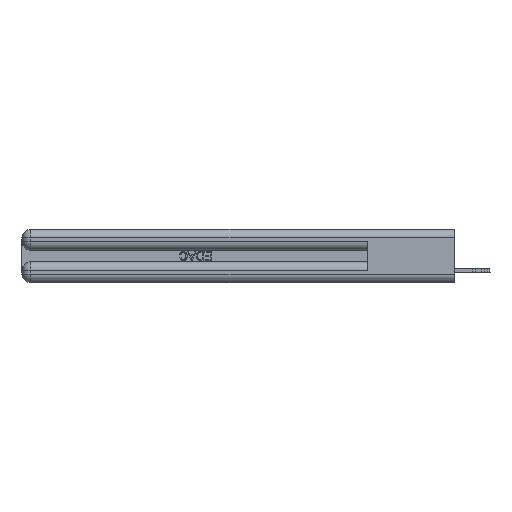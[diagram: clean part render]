
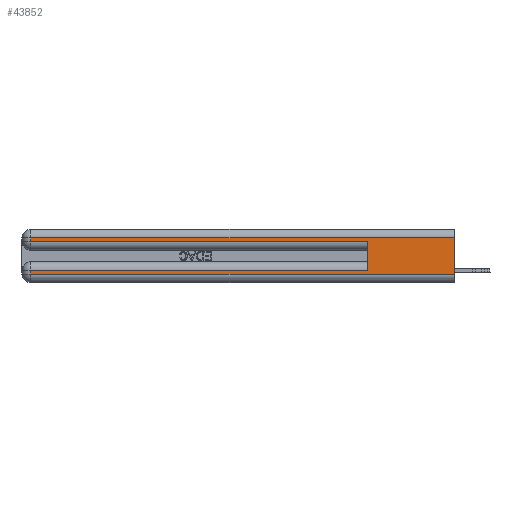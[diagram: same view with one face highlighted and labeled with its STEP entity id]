
A CAD part, left-side view. The second image highlights one B-rep face of the part: STEP entity #43852.
In plain terms, the highlighted planar face has unit normal (-1, 0, 0).
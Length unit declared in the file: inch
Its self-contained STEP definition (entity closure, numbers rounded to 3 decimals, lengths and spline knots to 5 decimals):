
#193 = VECTOR ( 'NONE', #38642, 39.37008 ) ;
#657 = VERTEX_POINT ( 'NONE', #24279 ) ;
#1644 = LINE ( 'NONE', #23310, #2255 ) ;
#1999 = VERTEX_POINT ( 'NONE', #6571 ) ;
#2255 = VECTOR ( 'NONE', #40804, 39.37008 ) ;
#2619 = ORIENTED_EDGE ( 'NONE', *, *, #31778, .T. ) ;
#2622 = VECTOR ( 'NONE', #15443, 39.37008 ) ;
#4887 = LINE ( 'NONE', #12556, #38072 ) ;
#5340 = EDGE_CURVE ( 'NONE', #1999, #20237, #39503, .T. ) ;
#5843 = ORIENTED_EDGE ( 'NONE', *, *, #5340, .T. ) ;
#6571 = CARTESIAN_POINT ( 'NONE',  ( 0., 2.94, 0.31 ) ) ;
#7212 = VERTEX_POINT ( 'NONE', #9270 ) ;
#8084 = LINE ( 'NONE', #36414, #35694 ) ;
#9270 = CARTESIAN_POINT ( 'NONE',  ( 0., 0., 0.06 ) ) ;
#10385 = AXIS2_PLACEMENT_3D ( 'NONE', #46592, #25127, #35892 ) ;
#10934 = DIRECTION ( 'NONE',  ( 0., 0., -1. ) ) ;
#12556 = CARTESIAN_POINT ( 'NONE',  ( 0., 0., 0.31 ) ) ;
#12734 = VERTEX_POINT ( 'NONE', #35527 ) ;
#13766 = LINE ( 'NONE', #38798, #193 ) ;
#14220 = PLANE ( 'NONE',  #10385 ) ;
#14344 = ORIENTED_EDGE ( 'NONE', *, *, #33568, .T. ) ;
#14900 = DIRECTION ( 'NONE',  ( 0., 1., 0. ) ) ;
#15334 = ORIENTED_EDGE ( 'NONE', *, *, #17748, .F. ) ;
#15363 = EDGE_CURVE ( 'NONE', #21128, #7212, #13766, .T. ) ;
#15443 = DIRECTION ( 'NONE',  ( 0., 0., -1. ) ) ;
#15903 = VECTOR ( 'NONE', #44245, 39.37008 ) ;
#17748 = EDGE_CURVE ( 'NONE', #12734, #657, #31736, .T. ) ;
#17859 = DIRECTION ( 'NONE',  ( 0., 0., 1. ) ) ;
#19142 = CARTESIAN_POINT ( 'NONE',  ( 0., 2.94, 0.37 ) ) ;
#20237 = VERTEX_POINT ( 'NONE', #33673 ) ;
#20327 = VECTOR ( 'NONE', #10934, 39.37008 ) ;
#20946 = EDGE_LOOP ( 'NONE', ( #27896, #14344, #5843, #44923, #15334, #2619, #46542, #33956 ) ) ;
#21128 = VERTEX_POINT ( 'NONE', #36643 ) ;
#22170 = VECTOR ( 'NONE', #17859, 39.37008 ) ;
#22489 = VERTEX_POINT ( 'NONE', #44840 ) ;
#23310 = CARTESIAN_POINT ( 'NONE',  ( 0., 0., 0.285 ) ) ;
#23622 = DIRECTION ( 'NONE',  ( 0., 1., 0. ) ) ;
#24279 = CARTESIAN_POINT ( 'NONE',  ( 0., 0.6, 0.285 ) ) ;
#25127 = DIRECTION ( 'NONE',  ( 1., 0., 0. ) ) ;
#25402 = CARTESIAN_POINT ( 'NONE',  ( 0., 0.6, 0.145 ) ) ;
#27673 = EDGE_CURVE ( 'NONE', #22489, #21128, #29817, .T. ) ;
#27896 = ORIENTED_EDGE ( 'NONE', *, *, #30560, .F. ) ;
#28928 = CARTESIAN_POINT ( 'NONE',  ( 0., 0., 0.31 ) ) ;
#29817 = LINE ( 'NONE', #31291, #20327 ) ;
#30062 = CARTESIAN_POINT ( 'NONE',  ( 0., 0., 0.37 ) ) ;
#30488 = FACE_OUTER_BOUND ( 'NONE', #20946, .T. ) ;
#30560 = EDGE_CURVE ( 'NONE', #37703, #7212, #40829, .T. ) ;
#31291 = CARTESIAN_POINT ( 'NONE',  ( 0., 2.94, 0.37 ) ) ;
#31736 = LINE ( 'NONE', #25402, #22170 ) ;
#31778 = EDGE_CURVE ( 'NONE', #12734, #22489, #8084, .T. ) ;
#33568 = EDGE_CURVE ( 'NONE', #37703, #1999, #4887, .T. ) ;
#33673 = CARTESIAN_POINT ( 'NONE',  ( 0., 2.94, 0.285 ) ) ;
#33956 = ORIENTED_EDGE ( 'NONE', *, *, #15363, .T. ) ;
#35527 = CARTESIAN_POINT ( 'NONE',  ( 0., 0.6, 0.085 ) ) ;
#35694 = VECTOR ( 'NONE', #14900, 39.37008 ) ;
#35892 = DIRECTION ( 'NONE',  ( 0., 0., -1. ) ) ;
#36414 = CARTESIAN_POINT ( 'NONE',  ( 0., 0., 0.085 ) ) ;
#36643 = CARTESIAN_POINT ( 'NONE',  ( 0., 2.94, 0.06 ) ) ;
#37703 = VERTEX_POINT ( 'NONE', #28928 ) ;
#38072 = VECTOR ( 'NONE', #23622, 39.37008 ) ;
#38642 = DIRECTION ( 'NONE',  ( 0., -1., 0. ) ) ;
#38798 = CARTESIAN_POINT ( 'NONE',  ( 0., 0., 0.06 ) ) ;
#39503 = LINE ( 'NONE', #19142, #15903 ) ;
#40804 = DIRECTION ( 'NONE',  ( 0., -1., 0. ) ) ;
#40829 = LINE ( 'NONE', #30062, #2622 ) ;
#43852 = ADVANCED_FACE ( 'NONE', ( #30488 ), #14220, .F. ) ;
#44245 = DIRECTION ( 'NONE',  ( 0., 0., -1. ) ) ;
#44762 = EDGE_CURVE ( 'NONE', #20237, #657, #1644, .T. ) ;
#44840 = CARTESIAN_POINT ( 'NONE',  ( 0., 2.94, 0.085 ) ) ;
#44923 = ORIENTED_EDGE ( 'NONE', *, *, #44762, .T. ) ;
#46542 = ORIENTED_EDGE ( 'NONE', *, *, #27673, .T. ) ;
#46592 = CARTESIAN_POINT ( 'NONE',  ( 0., 0., 0.37 ) ) ;
